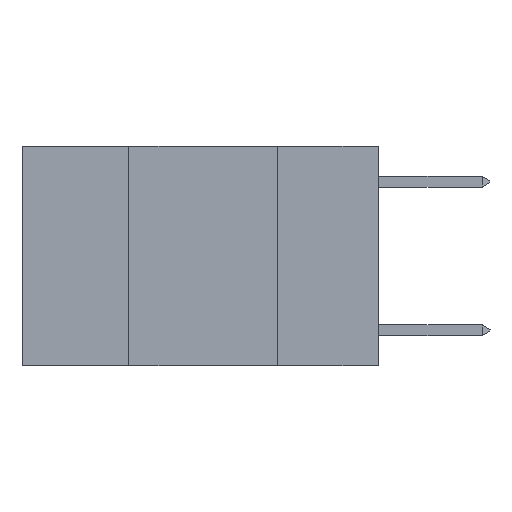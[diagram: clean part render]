
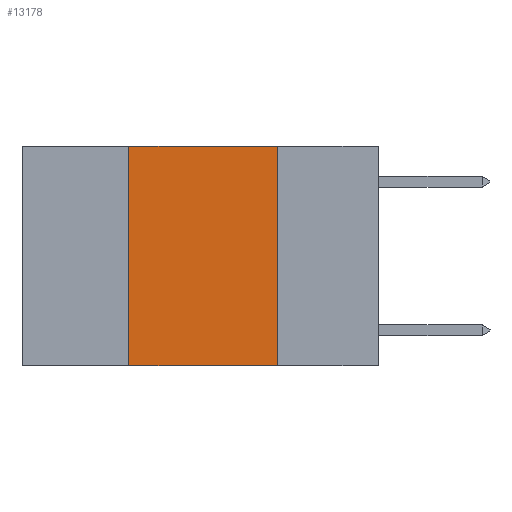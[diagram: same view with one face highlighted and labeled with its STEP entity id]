
A CAD part, left-side view. The second image highlights one B-rep face of the part: STEP entity #13178.
In plain terms, the highlighted planar face has unit normal (-1, 0, 0).
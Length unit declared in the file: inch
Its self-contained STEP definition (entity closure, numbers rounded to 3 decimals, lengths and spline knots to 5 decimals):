
#128 = PLANE ( 'NONE',  #17990 ) ;
#865 = ORIENTED_EDGE ( 'NONE', *, *, #24259, .F. ) ;
#944 = VERTEX_POINT ( 'NONE', #4930 ) ;
#2448 = VERTEX_POINT ( 'NONE', #11417 ) ;
#2859 = VECTOR ( 'NONE', #22068, 39.37008 ) ;
#3086 = DIRECTION ( 'NONE',  ( 0., 0., 1. ) ) ;
#3093 = LINE ( 'NONE', #20133, #2859 ) ;
#3506 = VECTOR ( 'NONE', #15478, 39.37008 ) ;
#3756 = LINE ( 'NONE', #13516, #3506 ) ;
#4930 = CARTESIAN_POINT ( 'NONE',  ( 0., 0.17, 0. ) ) ;
#6462 = VERTEX_POINT ( 'NONE', #23897 ) ;
#6898 = DIRECTION ( 'NONE',  ( 0., 0., -1. ) ) ;
#7727 = LINE ( 'NONE', #11268, #18007 ) ;
#8020 = ORIENTED_EDGE ( 'NONE', *, *, #15616, .F. ) ;
#9632 = EDGE_LOOP ( 'NONE', ( #865, #8020, #16714, #12941 ) ) ;
#11268 = CARTESIAN_POINT ( 'NONE',  ( 0., 0.17, 0. ) ) ;
#11417 = CARTESIAN_POINT ( 'NONE',  ( 0., 0.17, -0.37 ) ) ;
#12941 = ORIENTED_EDGE ( 'NONE', *, *, #21284, .T. ) ;
#13126 = FACE_OUTER_BOUND ( 'NONE', #9632, .T. ) ;
#13178 = ADVANCED_FACE ( 'NONE', ( #13126 ), #128, .F. ) ;
#13419 = DIRECTION ( 'NONE',  ( 0., 0., -1. ) ) ;
#13516 = CARTESIAN_POINT ( 'NONE',  ( 0., 0.6, -0.37 ) ) ;
#14656 = EDGE_CURVE ( 'NONE', #6462, #16648, #16424, .T. ) ;
#15214 = CARTESIAN_POINT ( 'NONE',  ( 0., 0.6, 0. ) ) ;
#15478 = DIRECTION ( 'NONE',  ( 0., -1., 0. ) ) ;
#15616 = EDGE_CURVE ( 'NONE', #16648, #944, #3093, .T. ) ;
#15706 = CARTESIAN_POINT ( 'NONE',  ( 0., 0.42, 0. ) ) ;
#16150 = VECTOR ( 'NONE', #3086, 39.37008 ) ;
#16424 = LINE ( 'NONE', #19735, #16150 ) ;
#16648 = VERTEX_POINT ( 'NONE', #15706 ) ;
#16714 = ORIENTED_EDGE ( 'NONE', *, *, #14656, .F. ) ;
#17990 = AXIS2_PLACEMENT_3D ( 'NONE', #15214, #19187, #6898 ) ;
#18007 = VECTOR ( 'NONE', #13419, 39.37008 ) ;
#19187 = DIRECTION ( 'NONE',  ( 1., 0., 0. ) ) ;
#19735 = CARTESIAN_POINT ( 'NONE',  ( 0., 0.42, 0. ) ) ;
#20133 = CARTESIAN_POINT ( 'NONE',  ( 0., 0.6, 0. ) ) ;
#21284 = EDGE_CURVE ( 'NONE', #6462, #2448, #3756, .T. ) ;
#22068 = DIRECTION ( 'NONE',  ( 0., -1., 0. ) ) ;
#23897 = CARTESIAN_POINT ( 'NONE',  ( 0., 0.42, -0.37 ) ) ;
#24259 = EDGE_CURVE ( 'NONE', #944, #2448, #7727, .T. ) ;
